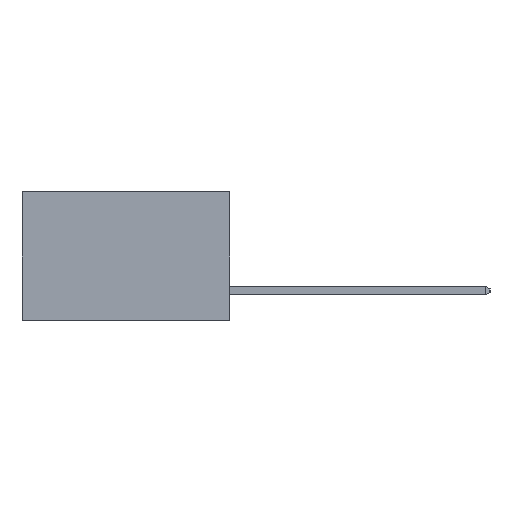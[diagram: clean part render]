
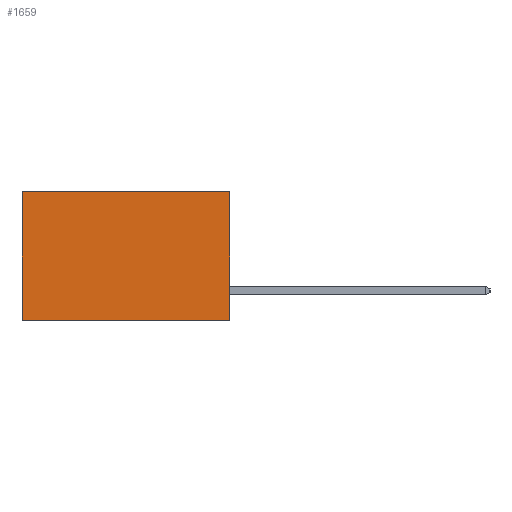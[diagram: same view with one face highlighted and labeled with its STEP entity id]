
A CAD part, left-side view. The second image highlights one B-rep face of the part: STEP entity #1659.
In plain terms, the highlighted planar face has unit normal (-1, 0, 0).
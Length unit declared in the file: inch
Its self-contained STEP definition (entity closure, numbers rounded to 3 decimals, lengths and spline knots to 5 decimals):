
#606 = EDGE_CURVE ( 'NONE', #1830, #1282, #3566, .T. ) ;
#1090 = ORIENTED_EDGE ( 'NONE', *, *, #606, .T. ) ;
#1282 = VERTEX_POINT ( 'NONE', #6425 ) ;
#1348 = DIRECTION ( 'NONE',  ( 0., 0., -1. ) ) ;
#1649 = AXIS2_PLACEMENT_3D ( 'NONE', #3971, #6761, #1348 ) ;
#1659 = ADVANCED_FACE ( 'NONE', ( #3336 ), #7217, .F. ) ;
#1675 = CARTESIAN_POINT ( 'NONE',  ( 0.2615, 0., -0.37 ) ) ;
#1682 = ORIENTED_EDGE ( 'NONE', *, *, #8494, .F. ) ;
#1796 = ORIENTED_EDGE ( 'NONE', *, *, #5130, .F. ) ;
#1830 = VERTEX_POINT ( 'NONE', #7364 ) ;
#2081 = VECTOR ( 'NONE', #2530, 39.37008 ) ;
#2084 = ORIENTED_EDGE ( 'NONE', *, *, #6262, .T. ) ;
#2159 = EDGE_LOOP ( 'NONE', ( #1090, #1682, #1796, #2084 ) ) ;
#2356 = DIRECTION ( 'NONE',  ( 0., 1., 0. ) ) ;
#2374 = CARTESIAN_POINT ( 'NONE',  ( 0.2615, 0., -0.37 ) ) ;
#2530 = DIRECTION ( 'NONE',  ( 0., 0., -1. ) ) ;
#3336 = FACE_OUTER_BOUND ( 'NONE', #2159, .T. ) ;
#3486 = VECTOR ( 'NONE', #8058, 39.37008 ) ;
#3566 = LINE ( 'NONE', #6142, #2081 ) ;
#3971 = CARTESIAN_POINT ( 'NONE',  ( 0.2615, 0., -0.37 ) ) ;
#5105 = LINE ( 'NONE', #2374, #6709 ) ;
#5130 = EDGE_CURVE ( 'NONE', #7075, #5795, #5923, .T. ) ;
#5551 = CARTESIAN_POINT ( 'NONE',  ( 0.2615, 0., -0.37 ) ) ;
#5589 = DIRECTION ( 'NONE',  ( 0., 0., -1. ) ) ;
#5795 = VERTEX_POINT ( 'NONE', #1675 ) ;
#5923 = LINE ( 'NONE', #5551, #7475 ) ;
#6142 = CARTESIAN_POINT ( 'NONE',  ( 0.2615, 0.6, -0.37 ) ) ;
#6181 = CARTESIAN_POINT ( 'NONE',  ( 0.2615, 0., 0. ) ) ;
#6262 = EDGE_CURVE ( 'NONE', #7075, #1830, #7149, .T. ) ;
#6425 = CARTESIAN_POINT ( 'NONE',  ( 0.2615, 0.6, -0.37 ) ) ;
#6709 = VECTOR ( 'NONE', #2356, 39.37008 ) ;
#6761 = DIRECTION ( 'NONE',  ( 1., 0., 0. ) ) ;
#7075 = VERTEX_POINT ( 'NONE', #6181 ) ;
#7149 = LINE ( 'NONE', #8126, #3486 ) ;
#7217 = PLANE ( 'NONE',  #1649 ) ;
#7364 = CARTESIAN_POINT ( 'NONE',  ( 0.2615, 0.6, 0. ) ) ;
#7475 = VECTOR ( 'NONE', #5589, 39.37008 ) ;
#8058 = DIRECTION ( 'NONE',  ( 0., 1., 0. ) ) ;
#8126 = CARTESIAN_POINT ( 'NONE',  ( 0.2615, 0., 0. ) ) ;
#8494 = EDGE_CURVE ( 'NONE', #5795, #1282, #5105, .T. ) ;
